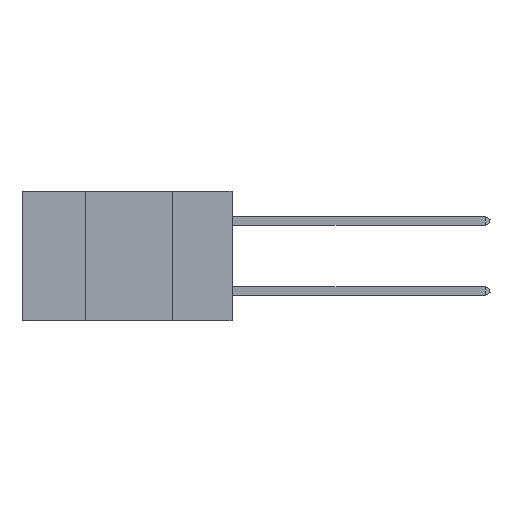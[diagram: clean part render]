
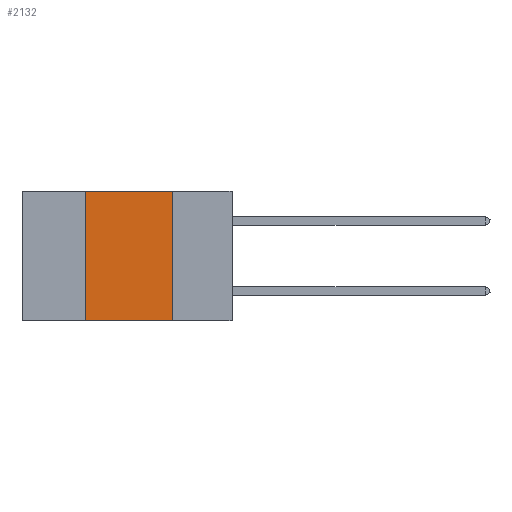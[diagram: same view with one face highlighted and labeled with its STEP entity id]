
A CAD part, left-side view. The second image highlights one B-rep face of the part: STEP entity #2132.
In plain terms, the highlighted planar face has unit normal (-1, 0, 0).
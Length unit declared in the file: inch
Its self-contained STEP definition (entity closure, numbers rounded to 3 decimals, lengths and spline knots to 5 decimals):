
#866 = ORIENTED_EDGE ( 'NONE', *, *, #37290, .F. ) ;
#2132 = ADVANCED_FACE ( 'NONE', ( #37045 ), #8188, .F. ) ;
#2906 = CARTESIAN_POINT ( 'NONE',  ( 0., 0.17, 0. ) ) ;
#8188 = PLANE ( 'NONE',  #28195 ) ;
#10845 = DIRECTION ( 'NONE',  ( 0., 0., 1. ) ) ;
#11420 = CARTESIAN_POINT ( 'NONE',  ( 0., 0.6, -0.37 ) ) ;
#11790 = DIRECTION ( 'NONE',  ( 1., 0., 0. ) ) ;
#12266 = CARTESIAN_POINT ( 'NONE',  ( 0., 0.17, 0. ) ) ;
#12420 = VERTEX_POINT ( 'NONE', #12266 ) ;
#12842 = VECTOR ( 'NONE', #34341, 39.37008 ) ;
#13208 = EDGE_LOOP ( 'NONE', ( #21205, #21591, #866, #25240 ) ) ;
#14163 = VERTEX_POINT ( 'NONE', #21871 ) ;
#17070 = EDGE_CURVE ( 'NONE', #12420, #29020, #18528, .T. ) ;
#18341 = CARTESIAN_POINT ( 'NONE',  ( 0., 0.42, 0. ) ) ;
#18528 = LINE ( 'NONE', #2906, #38834 ) ;
#18608 = DIRECTION ( 'NONE',  ( 0., -1., 0. ) ) ;
#20339 = DIRECTION ( 'NONE',  ( 0., 0., -1. ) ) ;
#20488 = CARTESIAN_POINT ( 'NONE',  ( 0., 0.6, 0. ) ) ;
#21205 = ORIENTED_EDGE ( 'NONE', *, *, #17070, .F. ) ;
#21591 = ORIENTED_EDGE ( 'NONE', *, *, #36042, .F. ) ;
#21871 = CARTESIAN_POINT ( 'NONE',  ( 0., 0.42, 0. ) ) ;
#22631 = DIRECTION ( 'NONE',  ( 0., 0., -1. ) ) ;
#25240 = ORIENTED_EDGE ( 'NONE', *, *, #34499, .T. ) ;
#26240 = CARTESIAN_POINT ( 'NONE',  ( 0., 0.17, -0.37 ) ) ;
#27585 = LINE ( 'NONE', #18341, #41144 ) ;
#28195 = AXIS2_PLACEMENT_3D ( 'NONE', #33305, #11790, #22631 ) ;
#29020 = VERTEX_POINT ( 'NONE', #26240 ) ;
#31385 = LINE ( 'NONE', #20488, #12842 ) ;
#33305 = CARTESIAN_POINT ( 'NONE',  ( 0., 0.6, 0. ) ) ;
#34266 = LINE ( 'NONE', #11420, #36539 ) ;
#34341 = DIRECTION ( 'NONE',  ( 0., -1., 0. ) ) ;
#34499 = EDGE_CURVE ( 'NONE', #39514, #29020, #34266, .T. ) ;
#36042 = EDGE_CURVE ( 'NONE', #14163, #12420, #31385, .T. ) ;
#36539 = VECTOR ( 'NONE', #18608, 39.37008 ) ;
#37045 = FACE_OUTER_BOUND ( 'NONE', #13208, .T. ) ;
#37290 = EDGE_CURVE ( 'NONE', #39514, #14163, #27585, .T. ) ;
#38834 = VECTOR ( 'NONE', #20339, 39.37008 ) ;
#39514 = VERTEX_POINT ( 'NONE', #44648 ) ;
#41144 = VECTOR ( 'NONE', #10845, 39.37008 ) ;
#44648 = CARTESIAN_POINT ( 'NONE',  ( 0., 0.42, -0.37 ) ) ;
